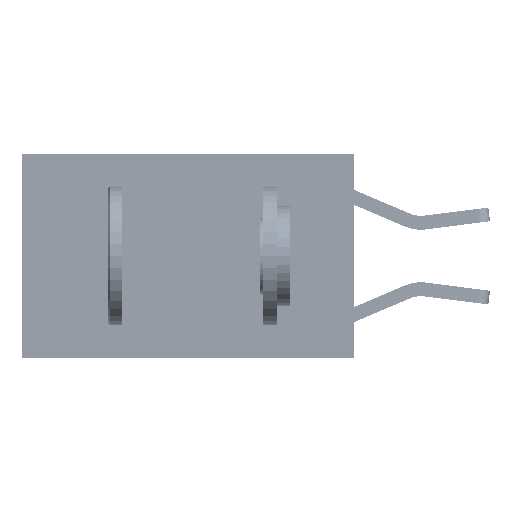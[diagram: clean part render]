
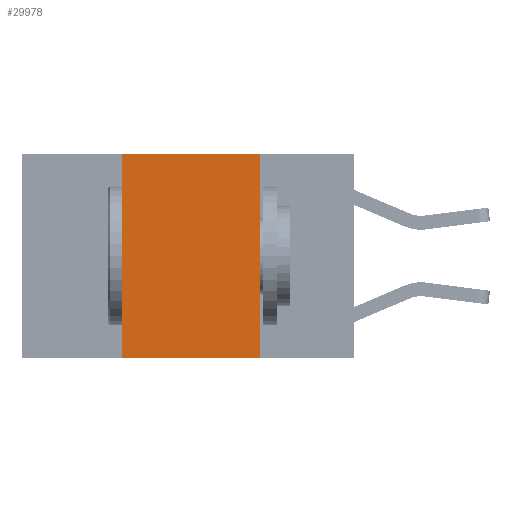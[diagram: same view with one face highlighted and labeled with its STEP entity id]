
A CAD part, left-side view. The second image highlights one B-rep face of the part: STEP entity #29978.
In plain terms, the highlighted planar face has unit normal (-1, 0, 0).
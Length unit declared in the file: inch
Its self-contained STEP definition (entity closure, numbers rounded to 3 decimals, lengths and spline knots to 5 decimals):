
#2012 = VERTEX_POINT ( 'NONE', #24683 ) ;
#2030 = CARTESIAN_POINT ( 'NONE',  ( 0., 0.6, -0.37 ) ) ;
#3331 = EDGE_CURVE ( 'NONE', #29550, #8209, #24075, .T. ) ;
#3626 = CARTESIAN_POINT ( 'NONE',  ( 0., 0.17, 0. ) ) ;
#3757 = CARTESIAN_POINT ( 'NONE',  ( 0., 0.6, 0. ) ) ;
#4025 = EDGE_CURVE ( 'NONE', #29550, #32408, #24422, .T. ) ;
#4096 = CARTESIAN_POINT ( 'NONE',  ( 0., 0.42, 0. ) ) ;
#4151 = ORIENTED_EDGE ( 'NONE', *, *, #12879, .F. ) ;
#4589 = CARTESIAN_POINT ( 'NONE',  ( 0., 0.17, -0.37 ) ) ;
#5053 = DIRECTION ( 'NONE',  ( 1., 0., 0. ) ) ;
#6793 = EDGE_CURVE ( 'NONE', #8209, #2012, #19208, .T. ) ;
#8209 = VERTEX_POINT ( 'NONE', #24990 ) ;
#8726 = DIRECTION ( 'NONE',  ( 0., 0., -1. ) ) ;
#9707 = DIRECTION ( 'NONE',  ( 0., -1., 0. ) ) ;
#10701 = VECTOR ( 'NONE', #21656, 39.37008 ) ;
#10895 = ORIENTED_EDGE ( 'NONE', *, *, #6793, .F. ) ;
#10963 = CARTESIAN_POINT ( 'NONE',  ( 0., 0.42, -0.37 ) ) ;
#12505 = VECTOR ( 'NONE', #23951, 39.37008 ) ;
#12879 = EDGE_CURVE ( 'NONE', #2012, #32408, #25690, .T. ) ;
#12902 = ORIENTED_EDGE ( 'NONE', *, *, #4025, .T. ) ;
#13109 = VECTOR ( 'NONE', #8726, 39.37008 ) ;
#18246 = AXIS2_PLACEMENT_3D ( 'NONE', #30186, #5053, #22699 ) ;
#19208 = LINE ( 'NONE', #3757, #12505 ) ;
#19496 = EDGE_LOOP ( 'NONE', ( #4151, #10895, #20747, #12902 ) ) ;
#20747 = ORIENTED_EDGE ( 'NONE', *, *, #3331, .F. ) ;
#21656 = DIRECTION ( 'NONE',  ( 0., 0., 1. ) ) ;
#22699 = DIRECTION ( 'NONE',  ( 0., 0., -1. ) ) ;
#23951 = DIRECTION ( 'NONE',  ( 0., -1., 0. ) ) ;
#24075 = LINE ( 'NONE', #4096, #10701 ) ;
#24422 = LINE ( 'NONE', #2030, #30338 ) ;
#24683 = CARTESIAN_POINT ( 'NONE',  ( 0., 0.17, 0. ) ) ;
#24990 = CARTESIAN_POINT ( 'NONE',  ( 0., 0.42, 0. ) ) ;
#25127 = PLANE ( 'NONE',  #18246 ) ;
#25623 = FACE_OUTER_BOUND ( 'NONE', #19496, .T. ) ;
#25690 = LINE ( 'NONE', #3626, #13109 ) ;
#29550 = VERTEX_POINT ( 'NONE', #10963 ) ;
#29978 = ADVANCED_FACE ( 'NONE', ( #25623 ), #25127, .F. ) ;
#30186 = CARTESIAN_POINT ( 'NONE',  ( 0., 0.6, 0. ) ) ;
#30338 = VECTOR ( 'NONE', #9707, 39.37008 ) ;
#32408 = VERTEX_POINT ( 'NONE', #4589 ) ;
